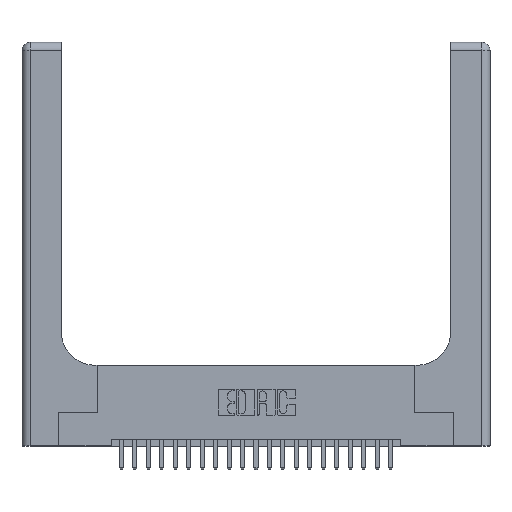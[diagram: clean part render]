
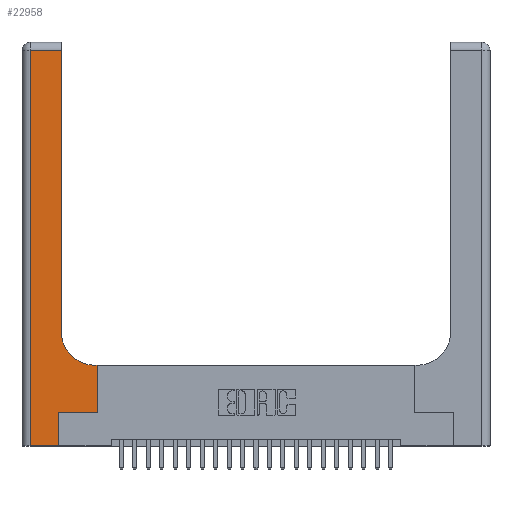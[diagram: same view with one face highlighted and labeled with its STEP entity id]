
A CAD part, top view. The second image highlights one B-rep face of the part: STEP entity #22958.
In plain terms, the highlighted planar face has unit normal (0, 0, 1).
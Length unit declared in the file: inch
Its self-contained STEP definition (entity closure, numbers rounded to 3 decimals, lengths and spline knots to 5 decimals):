
#331 = EDGE_CURVE ( 'NONE', #21988, #2618, #9742, .T. ) ;
#367 = ORIENTED_EDGE ( 'NONE', *, *, #18080, .T. ) ;
#575 = VERTEX_POINT ( 'NONE', #1232 ) ;
#858 = DIRECTION ( 'NONE',  ( -1., 0., 0. ) ) ;
#1053 = LINE ( 'NONE', #17867, #19741 ) ;
#1152 = EDGE_CURVE ( 'NONE', #23280, #21988, #23933, .T. ) ;
#1232 = CARTESIAN_POINT ( 'NONE',  ( 0.269, 0., 0.37 ) ) ;
#1279 = CIRCLE ( 'NONE', #2900, 0.25 ) ;
#1325 = DIRECTION ( 'NONE',  ( 0., -1., 0. ) ) ;
#1488 = VECTOR ( 'NONE', #1325, 39.37008 ) ;
#2377 = LINE ( 'NONE', #6511, #17502 ) ;
#2574 = CARTESIAN_POINT ( 'NONE',  ( 0.5585, 0.6, 0.37 ) ) ;
#2618 = VERTEX_POINT ( 'NONE', #2574 ) ;
#2634 = DIRECTION ( 'NONE',  ( 1., 0., 0. ) ) ;
#2900 = AXIS2_PLACEMENT_3D ( 'NONE', #11853, #13976, #2634 ) ;
#3734 = LINE ( 'NONE', #17494, #19405 ) ;
#3833 = EDGE_LOOP ( 'NONE', ( #7462, #9727, #367, #22209, #21589, #22765, #23119, #21651, #10310 ) ) ;
#4657 = EDGE_CURVE ( 'NONE', #5820, #5215, #2377, .T. ) ;
#4769 = CARTESIAN_POINT ( 'NONE',  ( 0.269, 0.25, 0.37 ) ) ;
#5215 = VERTEX_POINT ( 'NONE', #23010 ) ;
#5231 = CARTESIAN_POINT ( 'NONE',  ( 0.269, 0.25, 0.37 ) ) ;
#5496 = VECTOR ( 'NONE', #12139, 39.37008 ) ;
#5820 = VERTEX_POINT ( 'NONE', #13429 ) ;
#6310 = AXIS2_PLACEMENT_3D ( 'NONE', #19446, #6417, #23305 ) ;
#6417 = DIRECTION ( 'NONE',  ( 0., 0., -1. ) ) ;
#6511 = CARTESIAN_POINT ( 'NONE',  ( 0.2915, 3., 0.37 ) ) ;
#7462 = ORIENTED_EDGE ( 'NONE', *, *, #4657, .T. ) ;
#8592 = VERTEX_POINT ( 'NONE', #23575 ) ;
#8830 = DIRECTION ( 'NONE',  ( 1., 0., 0. ) ) ;
#9727 = ORIENTED_EDGE ( 'NONE', *, *, #23724, .T. ) ;
#9742 = LINE ( 'NONE', #21760, #20689 ) ;
#10023 = CARTESIAN_POINT ( 'NONE',  ( 0., 2.94, 0.37 ) ) ;
#10063 = VECTOR ( 'NONE', #858, 39.37008 ) ;
#10310 = ORIENTED_EDGE ( 'NONE', *, *, #20694, .T. ) ;
#10469 = EDGE_CURVE ( 'NONE', #2618, #16952, #1053, .T. ) ;
#10734 = LINE ( 'NONE', #15405, #1488 ) ;
#11085 = EDGE_CURVE ( 'NONE', #8592, #575, #23885, .T. ) ;
#11853 = CARTESIAN_POINT ( 'NONE',  ( 0.5415, 0.85, 0.37 ) ) ;
#12134 = CARTESIAN_POINT ( 'NONE',  ( 0.5415, 0.6, 0.37 ) ) ;
#12139 = DIRECTION ( 'NONE',  ( 1., 0., 0. ) ) ;
#13429 = CARTESIAN_POINT ( 'NONE',  ( 0.2915, 0.85, 0.37 ) ) ;
#13829 = VECTOR ( 'NONE', #8830, 39.37008 ) ;
#13976 = DIRECTION ( 'NONE',  ( 0., 0., -1. ) ) ;
#14676 = DIRECTION ( 'NONE',  ( 0., 1., 0. ) ) ;
#15069 = LINE ( 'NONE', #10023, #10063 ) ;
#15385 = CARTESIAN_POINT ( 'NONE',  ( 0.06, 2.94, 0.37 ) ) ;
#15405 = CARTESIAN_POINT ( 'NONE',  ( 0.06, 3., 0.37 ) ) ;
#15630 = EDGE_CURVE ( 'NONE', #575, #23280, #3734, .T. ) ;
#15861 = CARTESIAN_POINT ( 'NONE',  ( 0., 0., 0.37 ) ) ;
#16952 = VERTEX_POINT ( 'NONE', #12134 ) ;
#17254 = DIRECTION ( 'NONE',  ( 0., 1., 0. ) ) ;
#17494 = CARTESIAN_POINT ( 'NONE',  ( 0.269, 0., 0.37 ) ) ;
#17502 = VECTOR ( 'NONE', #23413, 39.37008 ) ;
#17867 = CARTESIAN_POINT ( 'NONE',  ( 0.2915, 0.6, 0.37 ) ) ;
#18080 = EDGE_CURVE ( 'NONE', #23512, #8592, #10734, .T. ) ;
#19405 = VECTOR ( 'NONE', #17254, 39.37008 ) ;
#19446 = CARTESIAN_POINT ( 'NONE',  ( 0., 3., 0.37 ) ) ;
#19590 = CARTESIAN_POINT ( 'NONE',  ( 0.5585, 0.25, 0.37 ) ) ;
#19741 = VECTOR ( 'NONE', #23615, 39.37008 ) ;
#20419 = FACE_OUTER_BOUND ( 'NONE', #3833, .T. ) ;
#20689 = VECTOR ( 'NONE', #14676, 39.37008 ) ;
#20694 = EDGE_CURVE ( 'NONE', #16952, #5820, #1279, .T. ) ;
#21589 = ORIENTED_EDGE ( 'NONE', *, *, #15630, .T. ) ;
#21651 = ORIENTED_EDGE ( 'NONE', *, *, #10469, .T. ) ;
#21760 = CARTESIAN_POINT ( 'NONE',  ( 0.5585, 0.25, 0.37 ) ) ;
#21988 = VERTEX_POINT ( 'NONE', #19590 ) ;
#22209 = ORIENTED_EDGE ( 'NONE', *, *, #11085, .T. ) ;
#22765 = ORIENTED_EDGE ( 'NONE', *, *, #1152, .T. ) ;
#22958 = ADVANCED_FACE ( 'NONE', ( #20419 ), #23227, .F. ) ;
#23010 = CARTESIAN_POINT ( 'NONE',  ( 0.2915, 2.94, 0.37 ) ) ;
#23119 = ORIENTED_EDGE ( 'NONE', *, *, #331, .T. ) ;
#23227 = PLANE ( 'NONE',  #6310 ) ;
#23280 = VERTEX_POINT ( 'NONE', #5231 ) ;
#23305 = DIRECTION ( 'NONE',  ( -1., 0., 0. ) ) ;
#23413 = DIRECTION ( 'NONE',  ( 0., 1., 0. ) ) ;
#23512 = VERTEX_POINT ( 'NONE', #15385 ) ;
#23575 = CARTESIAN_POINT ( 'NONE',  ( 0.06, 0., 0.37 ) ) ;
#23615 = DIRECTION ( 'NONE',  ( -1., 0., 0. ) ) ;
#23724 = EDGE_CURVE ( 'NONE', #5215, #23512, #15069, .T. ) ;
#23885 = LINE ( 'NONE', #15861, #5496 ) ;
#23933 = LINE ( 'NONE', #4769, #13829 ) ;
